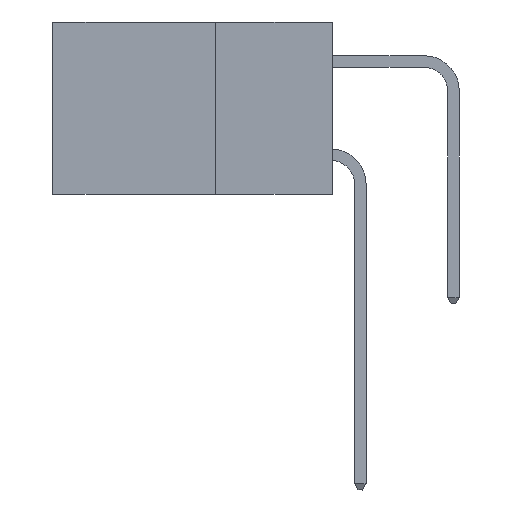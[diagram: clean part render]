
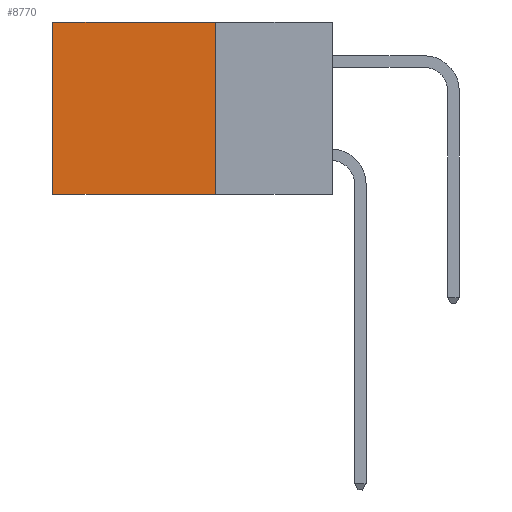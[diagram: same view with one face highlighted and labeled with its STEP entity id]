
A CAD part, left-side view. The second image highlights one B-rep face of the part: STEP entity #8770.
In plain terms, the highlighted planar face has unit normal (-1, 0, 0).
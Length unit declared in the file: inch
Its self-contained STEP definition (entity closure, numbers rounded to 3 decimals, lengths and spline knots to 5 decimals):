
#919 = VECTOR ( 'NONE', #4594, 39.37008 ) ;
#2261 = CARTESIAN_POINT ( 'NONE',  ( 0.298, 0.6, -0.37 ) ) ;
#2640 = VERTEX_POINT ( 'NONE', #2261 ) ;
#2884 = LINE ( 'NONE', #15990, #17557 ) ;
#4009 = VERTEX_POINT ( 'NONE', #25713 ) ;
#4156 = ORIENTED_EDGE ( 'NONE', *, *, #13137, .F. ) ;
#4207 = EDGE_LOOP ( 'NONE', ( #20957, #4156, #30355, #9258 ) ) ;
#4594 = DIRECTION ( 'NONE',  ( 0., 0., -1. ) ) ;
#4841 = CARTESIAN_POINT ( 'NONE',  ( 0.298, 0.25, 0. ) ) ;
#5140 = LINE ( 'NONE', #4841, #18637 ) ;
#5351 = LINE ( 'NONE', #23837, #20439 ) ;
#5727 = CARTESIAN_POINT ( 'NONE',  ( 0.298, 0.25, -0.37 ) ) ;
#5883 = DIRECTION ( 'NONE',  ( 0., 0., -1. ) ) ;
#6398 = CARTESIAN_POINT ( 'NONE',  ( 0.298, 0.6, 0. ) ) ;
#8770 = ADVANCED_FACE ( 'NONE', ( #24712 ), #18904, .F. ) ;
#9087 = VERTEX_POINT ( 'NONE', #5727 ) ;
#9202 = VERTEX_POINT ( 'NONE', #6398 ) ;
#9258 = ORIENTED_EDGE ( 'NONE', *, *, #9527, .T. ) ;
#9527 = EDGE_CURVE ( 'NONE', #4009, #9202, #5140, .T. ) ;
#10110 = DIRECTION ( 'NONE',  ( 0., 1., 0. ) ) ;
#13137 = EDGE_CURVE ( 'NONE', #9087, #2640, #2884, .T. ) ;
#14404 = LINE ( 'NONE', #19882, #919 ) ;
#15990 = CARTESIAN_POINT ( 'NONE',  ( 0.298, 0.25, -0.37 ) ) ;
#17557 = VECTOR ( 'NONE', #21197, 39.37008 ) ;
#18637 = VECTOR ( 'NONE', #10110, 39.37008 ) ;
#18862 = DIRECTION ( 'NONE',  ( 0., 0., -1. ) ) ;
#18904 = PLANE ( 'NONE',  #32652 ) ;
#19112 = DIRECTION ( 'NONE',  ( 1., 0., 0. ) ) ;
#19551 = EDGE_CURVE ( 'NONE', #9202, #2640, #14404, .T. ) ;
#19882 = CARTESIAN_POINT ( 'NONE',  ( 0.298, 0.6, 0. ) ) ;
#20439 = VECTOR ( 'NONE', #18862, 39.37008 ) ;
#20957 = ORIENTED_EDGE ( 'NONE', *, *, #19551, .T. ) ;
#21197 = DIRECTION ( 'NONE',  ( 0., 1., 0. ) ) ;
#23837 = CARTESIAN_POINT ( 'NONE',  ( 0.298, 0.25, 0. ) ) ;
#24428 = CARTESIAN_POINT ( 'NONE',  ( 0.298, 0.25, 0. ) ) ;
#24712 = FACE_OUTER_BOUND ( 'NONE', #4207, .T. ) ;
#25713 = CARTESIAN_POINT ( 'NONE',  ( 0.298, 0.25, 0. ) ) ;
#30355 = ORIENTED_EDGE ( 'NONE', *, *, #31703, .F. ) ;
#31703 = EDGE_CURVE ( 'NONE', #4009, #9087, #5351, .T. ) ;
#32652 = AXIS2_PLACEMENT_3D ( 'NONE', #24428, #19112, #5883 ) ;
